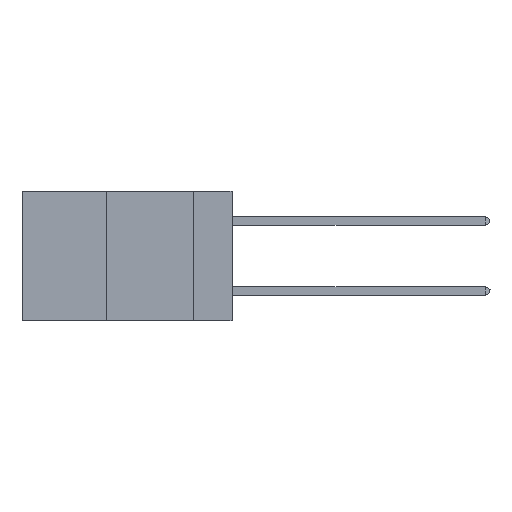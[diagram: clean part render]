
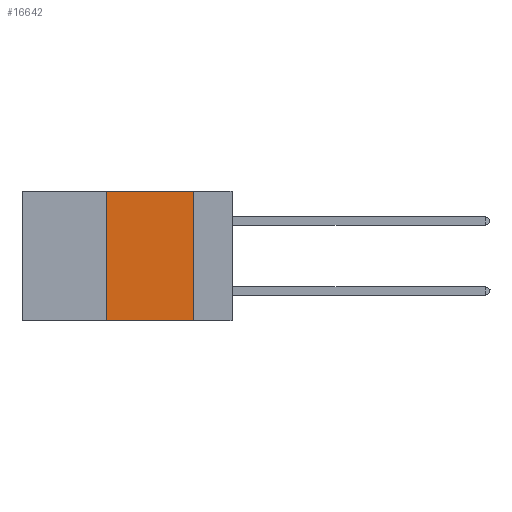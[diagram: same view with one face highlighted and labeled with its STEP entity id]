
A CAD part, left-side view. The second image highlights one B-rep face of the part: STEP entity #16642.
In plain terms, the highlighted planar face has unit normal (-1, 0, 0).
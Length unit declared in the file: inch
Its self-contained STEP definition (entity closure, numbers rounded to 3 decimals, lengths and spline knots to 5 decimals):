
#105 = VECTOR ( 'NONE', #11873, 39.37008 ) ;
#117 = VECTOR ( 'NONE', #4372, 39.37008 ) ;
#982 = PLANE ( 'NONE',  #13979 ) ;
#2333 = EDGE_CURVE ( 'NONE', #17800, #17323, #5476, .T. ) ;
#2671 = VECTOR ( 'NONE', #16453, 39.37008 ) ;
#2909 = VECTOR ( 'NONE', #10554, 39.37008 ) ;
#3507 = LINE ( 'NONE', #10871, #2671 ) ;
#3519 = LINE ( 'NONE', #9400, #2909 ) ;
#3571 = EDGE_LOOP ( 'NONE', ( #10750, #9748, #17624, #13231 ) ) ;
#4372 = DIRECTION ( 'NONE',  ( 0., -1., 0. ) ) ;
#5191 = CARTESIAN_POINT ( 'NONE',  ( 0., 0.11, 0. ) ) ;
#5476 = LINE ( 'NONE', #17201, #105 ) ;
#6663 = CARTESIAN_POINT ( 'NONE',  ( 0., 0.36, -0.37 ) ) ;
#6724 = CARTESIAN_POINT ( 'NONE',  ( 0., 0.11, -0.37 ) ) ;
#7778 = FACE_OUTER_BOUND ( 'NONE', #3571, .T. ) ;
#8197 = DIRECTION ( 'NONE',  ( 1., 0., 0. ) ) ;
#8248 = EDGE_CURVE ( 'NONE', #8377, #17828, #3519, .T. ) ;
#8377 = VERTEX_POINT ( 'NONE', #6663 ) ;
#8415 = EDGE_CURVE ( 'NONE', #17828, #17800, #3507, .T. ) ;
#9400 = CARTESIAN_POINT ( 'NONE',  ( 0., 0.36, 0. ) ) ;
#9748 = ORIENTED_EDGE ( 'NONE', *, *, #8415, .F. ) ;
#10554 = DIRECTION ( 'NONE',  ( 0., 0., 1. ) ) ;
#10750 = ORIENTED_EDGE ( 'NONE', *, *, #2333, .F. ) ;
#10832 = DIRECTION ( 'NONE',  ( 0., 0., -1. ) ) ;
#10871 = CARTESIAN_POINT ( 'NONE',  ( 0., 0.6, 0. ) ) ;
#11734 = EDGE_CURVE ( 'NONE', #8377, #17323, #11813, .T. ) ;
#11813 = LINE ( 'NONE', #14054, #117 ) ;
#11873 = DIRECTION ( 'NONE',  ( 0., 0., -1. ) ) ;
#13231 = ORIENTED_EDGE ( 'NONE', *, *, #11734, .T. ) ;
#13627 = CARTESIAN_POINT ( 'NONE',  ( 0., 0.6, 0. ) ) ;
#13979 = AXIS2_PLACEMENT_3D ( 'NONE', #13627, #8197, #10832 ) ;
#14054 = CARTESIAN_POINT ( 'NONE',  ( 0., 0.6, -0.37 ) ) ;
#15013 = CARTESIAN_POINT ( 'NONE',  ( 0., 0.36, 0. ) ) ;
#16453 = DIRECTION ( 'NONE',  ( 0., -1., 0. ) ) ;
#16642 = ADVANCED_FACE ( 'NONE', ( #7778 ), #982, .F. ) ;
#17201 = CARTESIAN_POINT ( 'NONE',  ( 0., 0.11, 0. ) ) ;
#17323 = VERTEX_POINT ( 'NONE', #6724 ) ;
#17624 = ORIENTED_EDGE ( 'NONE', *, *, #8248, .F. ) ;
#17800 = VERTEX_POINT ( 'NONE', #5191 ) ;
#17828 = VERTEX_POINT ( 'NONE', #15013 ) ;
